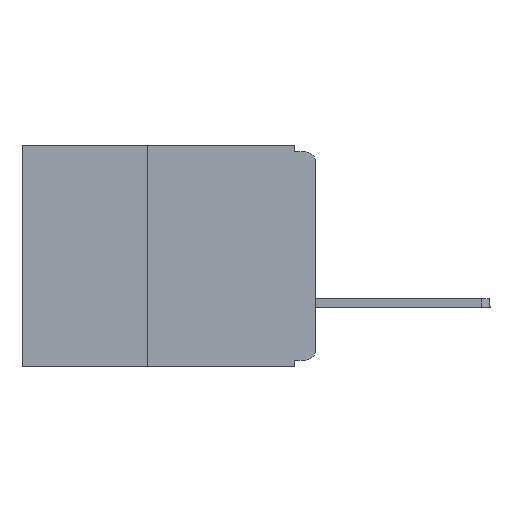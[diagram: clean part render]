
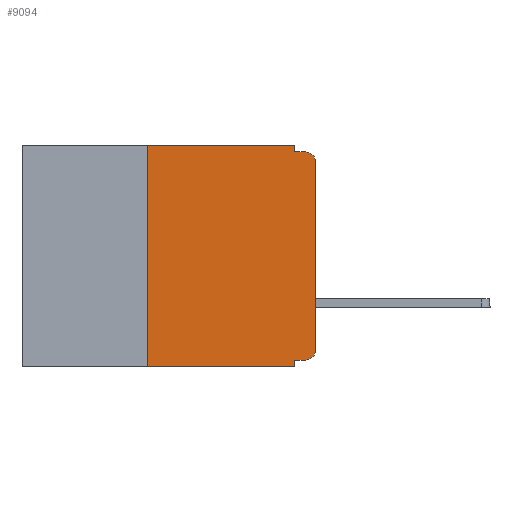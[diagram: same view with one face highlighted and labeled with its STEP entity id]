
A CAD part, left-side view. The second image highlights one B-rep face of the part: STEP entity #9094.
In plain terms, the highlighted planar face has unit normal (-1, 0, 0).
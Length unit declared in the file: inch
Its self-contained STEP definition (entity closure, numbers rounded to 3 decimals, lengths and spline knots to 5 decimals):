
#981 = FACE_OUTER_BOUND ( 'NONE', #11067, .T. ) ;
#1088 = CARTESIAN_POINT ( 'NONE',  ( 0., 0.031, -0.33 ) ) ;
#1387 = CARTESIAN_POINT ( 'NONE',  ( 0., 0.015, -0.025 ) ) ;
#1575 = EDGE_CURVE ( 'NONE', #1789, #9268, #16648, .T. ) ;
#1788 = ORIENTED_EDGE ( 'NONE', *, *, #15955, .F. ) ;
#1789 = VERTEX_POINT ( 'NONE', #10667 ) ;
#1867 = VECTOR ( 'NONE', #9457, 39.37008 ) ;
#1946 = CARTESIAN_POINT ( 'NONE',  ( 0., 0., -0.305 ) ) ;
#1970 = LINE ( 'NONE', #10531, #1867 ) ;
#2049 = VECTOR ( 'NONE', #13529, 39.37008 ) ;
#2089 = LINE ( 'NONE', #13722, #2049 ) ;
#2169 = ORIENTED_EDGE ( 'NONE', *, *, #12937, .F. ) ;
#2430 = CARTESIAN_POINT ( 'NONE',  ( 0., 0.031, -0.32 ) ) ;
#2603 = VECTOR ( 'NONE', #12352, 39.37008 ) ;
#2717 = VERTEX_POINT ( 'NONE', #6287 ) ;
#2963 = DIRECTION ( 'NONE',  ( -1., 0., 0. ) ) ;
#3030 = LINE ( 'NONE', #13780, #2603 ) ;
#3050 = EDGE_CURVE ( 'NONE', #15910, #5269, #7868, .T. ) ;
#3764 = VERTEX_POINT ( 'NONE', #1946 ) ;
#3826 = ORIENTED_EDGE ( 'NONE', *, *, #16148, .T. ) ;
#3968 = EDGE_CURVE ( 'NONE', #2717, #16254, #4207, .T. ) ;
#3994 = DIRECTION ( 'NONE',  ( 0., -1., 0. ) ) ;
#4061 = CARTESIAN_POINT ( 'NONE',  ( 0., 0., -0.01 ) ) ;
#4183 = VECTOR ( 'NONE', #6239, 39.37008 ) ;
#4207 = LINE ( 'NONE', #14461, #4183 ) ;
#4735 = VECTOR ( 'NONE', #14566, 39.37008 ) ;
#5036 = LINE ( 'NONE', #13059, #4735 ) ;
#5111 = EDGE_CURVE ( 'NONE', #1789, #3764, #18053, .T. ) ;
#5269 = VERTEX_POINT ( 'NONE', #5303 ) ;
#5303 = CARTESIAN_POINT ( 'NONE',  ( 0., 0.015, -0.01 ) ) ;
#5368 = VERTEX_POINT ( 'NONE', #1088 ) ;
#6205 = CARTESIAN_POINT ( 'NONE',  ( 0., 0.25, -0.33 ) ) ;
#6239 = DIRECTION ( 'NONE',  ( 0., 0., -1. ) ) ;
#6287 = CARTESIAN_POINT ( 'NONE',  ( 0., 0.031, 0. ) ) ;
#7235 = ORIENTED_EDGE ( 'NONE', *, *, #16296, .F. ) ;
#7563 = AXIS2_PLACEMENT_3D ( 'NONE', #14816, #14253, #14199 ) ;
#7868 = CIRCLE ( 'NONE', #15541, 0.015 ) ;
#8070 = ORIENTED_EDGE ( 'NONE', *, *, #17970, .F. ) ;
#8115 = DIRECTION ( 'NONE',  ( 0., 0., -1. ) ) ;
#8596 = VECTOR ( 'NONE', #3994, 39.37008 ) ;
#8653 = LINE ( 'NONE', #4061, #8596 ) ;
#8657 = VERTEX_POINT ( 'NONE', #6205 ) ;
#9094 = ADVANCED_FACE ( 'NONE', ( #981 ), #14351, .F. ) ;
#9202 = VECTOR ( 'NONE', #15635, 39.37008 ) ;
#9227 = LINE ( 'NONE', #15332, #9202 ) ;
#9268 = VERTEX_POINT ( 'NONE', #2430 ) ;
#9330 = ORIENTED_EDGE ( 'NONE', *, *, #3968, .F. ) ;
#9338 = ORIENTED_EDGE ( 'NONE', *, *, #1575, .F. ) ;
#9457 = DIRECTION ( 'NONE',  ( 0., 0., -1. ) ) ;
#10531 = CARTESIAN_POINT ( 'NONE',  ( 0., 0.031, -0.33 ) ) ;
#10667 = CARTESIAN_POINT ( 'NONE',  ( 0., 0.015, -0.32 ) ) ;
#11067 = EDGE_LOOP ( 'NONE', ( #11856, #12522, #8070, #9330, #2169, #1788, #3826, #7235, #9338, #12490 ) ) ;
#11084 = DIRECTION ( 'NONE',  ( 0., 1., 0. ) ) ;
#11226 = CARTESIAN_POINT ( 'NONE',  ( 0., 0., -0.32 ) ) ;
#11714 = AXIS2_PLACEMENT_3D ( 'NONE', #12489, #12432, #12254 ) ;
#11856 = ORIENTED_EDGE ( 'NONE', *, *, #16246, .T. ) ;
#12254 = DIRECTION ( 'NONE',  ( 0., 0., -1. ) ) ;
#12352 = DIRECTION ( 'NONE',  ( 0., -1., 0. ) ) ;
#12432 = DIRECTION ( 'NONE',  ( -1., 0., 0. ) ) ;
#12489 = CARTESIAN_POINT ( 'NONE',  ( 0., 0.015, -0.305 ) ) ;
#12490 = ORIENTED_EDGE ( 'NONE', *, *, #5111, .T. ) ;
#12522 = ORIENTED_EDGE ( 'NONE', *, *, #3050, .T. ) ;
#12937 = EDGE_CURVE ( 'NONE', #14428, #2717, #9227, .T. ) ;
#13059 = CARTESIAN_POINT ( 'NONE',  ( 0., 0.25, -0.33 ) ) ;
#13529 = DIRECTION ( 'NONE',  ( 0., 0., 1. ) ) ;
#13722 = CARTESIAN_POINT ( 'NONE',  ( 0., 0., 0. ) ) ;
#13780 = CARTESIAN_POINT ( 'NONE',  ( 0., 0.437, -0.33 ) ) ;
#14199 = DIRECTION ( 'NONE',  ( 0., 0., -1. ) ) ;
#14253 = DIRECTION ( 'NONE',  ( 1., 0., 0. ) ) ;
#14351 = PLANE ( 'NONE',  #7563 ) ;
#14428 = VERTEX_POINT ( 'NONE', #15970 ) ;
#14461 = CARTESIAN_POINT ( 'NONE',  ( 0., 0.031, 0. ) ) ;
#14566 = DIRECTION ( 'NONE',  ( 0., 0., 1. ) ) ;
#14649 = CARTESIAN_POINT ( 'NONE',  ( 0., 0.031, -0.01 ) ) ;
#14816 = CARTESIAN_POINT ( 'NONE',  ( 0., 0.437, 0. ) ) ;
#15332 = CARTESIAN_POINT ( 'NONE',  ( 0., 0.437, 0. ) ) ;
#15541 = AXIS2_PLACEMENT_3D ( 'NONE', #1387, #2963, #8115 ) ;
#15635 = DIRECTION ( 'NONE',  ( 0., -1., 0. ) ) ;
#15910 = VERTEX_POINT ( 'NONE', #18336 ) ;
#15955 = EDGE_CURVE ( 'NONE', #8657, #14428, #5036, .T. ) ;
#15970 = CARTESIAN_POINT ( 'NONE',  ( 0., 0.25, 0. ) ) ;
#16148 = EDGE_CURVE ( 'NONE', #8657, #5368, #3030, .T. ) ;
#16246 = EDGE_CURVE ( 'NONE', #3764, #15910, #2089, .T. ) ;
#16254 = VERTEX_POINT ( 'NONE', #14649 ) ;
#16296 = EDGE_CURVE ( 'NONE', #9268, #5368, #1970, .T. ) ;
#16648 = LINE ( 'NONE', #11226, #16688 ) ;
#16688 = VECTOR ( 'NONE', #11084, 39.37008 ) ;
#17970 = EDGE_CURVE ( 'NONE', #16254, #5269, #8653, .T. ) ;
#18053 = CIRCLE ( 'NONE', #11714, 0.015 ) ;
#18336 = CARTESIAN_POINT ( 'NONE',  ( 0., 0., -0.025 ) ) ;
